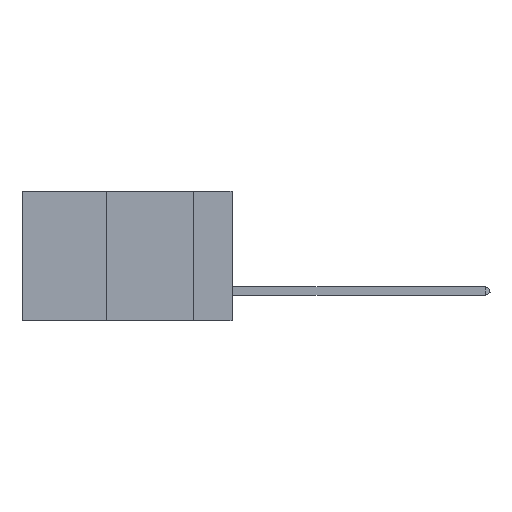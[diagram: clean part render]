
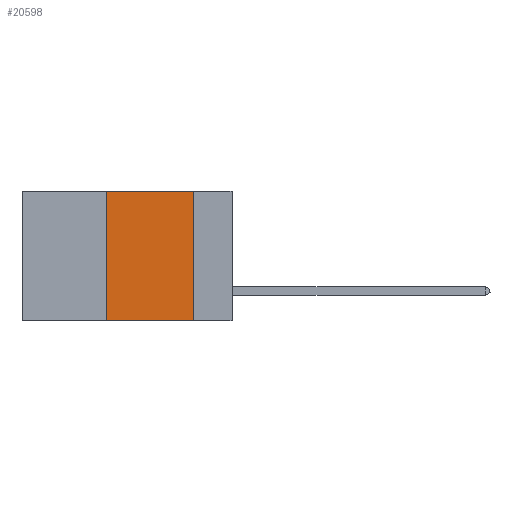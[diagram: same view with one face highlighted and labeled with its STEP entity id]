
A CAD part, left-side view. The second image highlights one B-rep face of the part: STEP entity #20598.
In plain terms, the highlighted planar face has unit normal (-1, 0, 0).
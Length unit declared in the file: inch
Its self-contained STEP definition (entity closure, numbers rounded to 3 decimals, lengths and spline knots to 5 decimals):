
#375 = EDGE_CURVE ( 'NONE', #11693, #7635, #15717, .T. ) ;
#1195 = VECTOR ( 'NONE', #12518, 39.37008 ) ;
#1475 = DIRECTION ( 'NONE',  ( 0., -1., 0. ) ) ;
#1670 = CARTESIAN_POINT ( 'NONE',  ( 0., 0.11, 0. ) ) ;
#2133 = AXIS2_PLACEMENT_3D ( 'NONE', #9626, #6114, #7963 ) ;
#2954 = ORIENTED_EDGE ( 'NONE', *, *, #11101, .F. ) ;
#3865 = LINE ( 'NONE', #15647, #1195 ) ;
#4557 = DIRECTION ( 'NONE',  ( 0., -1., 0. ) ) ;
#4754 = VECTOR ( 'NONE', #1475, 39.37008 ) ;
#5796 = VERTEX_POINT ( 'NONE', #6778 ) ;
#6023 = CARTESIAN_POINT ( 'NONE',  ( 0., 0.36, -0.37 ) ) ;
#6114 = DIRECTION ( 'NONE',  ( 1., 0., 0. ) ) ;
#6778 = CARTESIAN_POINT ( 'NONE',  ( 0., 0.11, -0.37 ) ) ;
#6929 = VECTOR ( 'NONE', #20987, 39.37008 ) ;
#7635 = VERTEX_POINT ( 'NONE', #1670 ) ;
#7963 = DIRECTION ( 'NONE',  ( 0., 0., -1. ) ) ;
#8004 = CARTESIAN_POINT ( 'NONE',  ( 0., 0.6, -0.37 ) ) ;
#9626 = CARTESIAN_POINT ( 'NONE',  ( 0., 0.6, 0. ) ) ;
#10231 = LINE ( 'NONE', #22505, #6929 ) ;
#10410 = FACE_OUTER_BOUND ( 'NONE', #13640, .T. ) ;
#10853 = ORIENTED_EDGE ( 'NONE', *, *, #17225, .F. ) ;
#11101 = EDGE_CURVE ( 'NONE', #7635, #5796, #3865, .T. ) ;
#11190 = ORIENTED_EDGE ( 'NONE', *, *, #15985, .T. ) ;
#11482 = PLANE ( 'NONE',  #2133 ) ;
#11693 = VERTEX_POINT ( 'NONE', #13344 ) ;
#12518 = DIRECTION ( 'NONE',  ( 0., 0., -1. ) ) ;
#13344 = CARTESIAN_POINT ( 'NONE',  ( 0., 0.36, 0. ) ) ;
#13640 = EDGE_LOOP ( 'NONE', ( #2954, #15638, #10853, #11190 ) ) ;
#14110 = VECTOR ( 'NONE', #4557, 39.37008 ) ;
#14771 = VERTEX_POINT ( 'NONE', #6023 ) ;
#15638 = ORIENTED_EDGE ( 'NONE', *, *, #375, .F. ) ;
#15647 = CARTESIAN_POINT ( 'NONE',  ( 0., 0.11, 0. ) ) ;
#15717 = LINE ( 'NONE', #17273, #4754 ) ;
#15985 = EDGE_CURVE ( 'NONE', #14771, #5796, #17364, .T. ) ;
#17225 = EDGE_CURVE ( 'NONE', #14771, #11693, #10231, .T. ) ;
#17273 = CARTESIAN_POINT ( 'NONE',  ( 0., 0.6, 0. ) ) ;
#17364 = LINE ( 'NONE', #8004, #14110 ) ;
#20598 = ADVANCED_FACE ( 'NONE', ( #10410 ), #11482, .F. ) ;
#20987 = DIRECTION ( 'NONE',  ( 0., 0., 1. ) ) ;
#22505 = CARTESIAN_POINT ( 'NONE',  ( 0., 0.36, 0. ) ) ;
